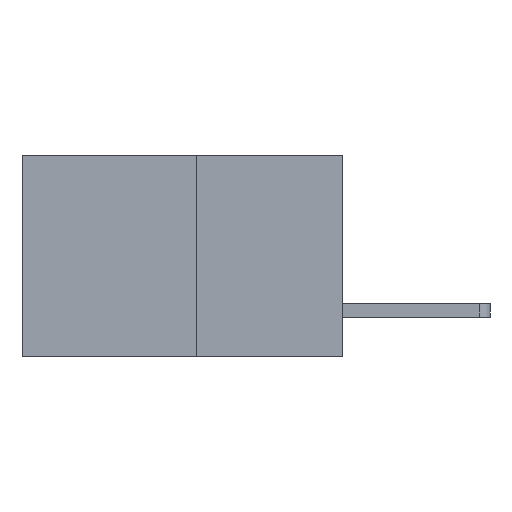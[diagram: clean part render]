
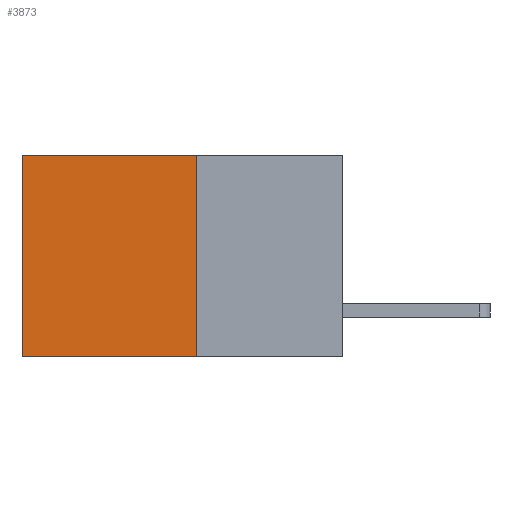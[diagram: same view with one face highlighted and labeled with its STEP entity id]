
A CAD part, left-side view. The second image highlights one B-rep face of the part: STEP entity #3873.
In plain terms, the highlighted planar face has unit normal (-1, 0, 0).
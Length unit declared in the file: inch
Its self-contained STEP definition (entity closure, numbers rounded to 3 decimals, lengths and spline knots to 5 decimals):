
#268 = VERTEX_POINT ( 'NONE', #2553 ) ;
#429 = LINE ( 'NONE', #6060, #4109 ) ;
#767 = LINE ( 'NONE', #8134, #6339 ) ;
#948 = ORIENTED_EDGE ( 'NONE', *, *, #2649, .T. ) ;
#991 = VECTOR ( 'NONE', #4728, 39.37008 ) ;
#1065 = ORIENTED_EDGE ( 'NONE', *, *, #2760, .T. ) ;
#1213 = ORIENTED_EDGE ( 'NONE', *, *, #8194, .F. ) ;
#1446 = VERTEX_POINT ( 'NONE', #3208 ) ;
#1551 = LINE ( 'NONE', #8164, #8953 ) ;
#2466 = EDGE_CURVE ( 'NONE', #268, #2572, #1551, .T. ) ;
#2553 = CARTESIAN_POINT ( 'NONE',  ( 0.277, 0.27, 0. ) ) ;
#2572 = VERTEX_POINT ( 'NONE', #7183 ) ;
#2649 = EDGE_CURVE ( 'NONE', #268, #1446, #429, .T. ) ;
#2760 = EDGE_CURVE ( 'NONE', #1446, #2761, #6790, .T. ) ;
#2761 = VERTEX_POINT ( 'NONE', #4672 ) ;
#3208 = CARTESIAN_POINT ( 'NONE',  ( 0.277, 0.59, 0. ) ) ;
#3741 = ORIENTED_EDGE ( 'NONE', *, *, #2466, .F. ) ;
#3873 = ADVANCED_FACE ( 'NONE', ( #4999 ), #4704, .F. ) ;
#3883 = DIRECTION ( 'NONE',  ( 0., 1., 0. ) ) ;
#4109 = VECTOR ( 'NONE', #6107, 39.37008 ) ;
#4413 = DIRECTION ( 'NONE',  ( 0., 0., -1. ) ) ;
#4636 = DIRECTION ( 'NONE',  ( 1., 0., 0. ) ) ;
#4670 = CARTESIAN_POINT ( 'NONE',  ( 0.277, 0.27, -0.37 ) ) ;
#4672 = CARTESIAN_POINT ( 'NONE',  ( 0.277, 0.59, -0.37 ) ) ;
#4682 = CARTESIAN_POINT ( 'NONE',  ( 0.277, 0.59, -0.37 ) ) ;
#4697 = AXIS2_PLACEMENT_3D ( 'NONE', #4670, #4636, #4413 ) ;
#4704 = PLANE ( 'NONE',  #4697 ) ;
#4728 = DIRECTION ( 'NONE',  ( 0., 0., -1. ) ) ;
#4845 = EDGE_LOOP ( 'NONE', ( #1065, #1213, #3741, #948 ) ) ;
#4999 = FACE_OUTER_BOUND ( 'NONE', #4845, .T. ) ;
#6060 = CARTESIAN_POINT ( 'NONE',  ( 0.277, 0.27, 0. ) ) ;
#6107 = DIRECTION ( 'NONE',  ( 0., 1., 0. ) ) ;
#6339 = VECTOR ( 'NONE', #3883, 39.37008 ) ;
#6790 = LINE ( 'NONE', #4682, #991 ) ;
#7183 = CARTESIAN_POINT ( 'NONE',  ( 0.277, 0.27, -0.37 ) ) ;
#7360 = DIRECTION ( 'NONE',  ( 0., 0., -1. ) ) ;
#8134 = CARTESIAN_POINT ( 'NONE',  ( 0.277, 0.27, -0.37 ) ) ;
#8164 = CARTESIAN_POINT ( 'NONE',  ( 0.277, 0.27, -0.37 ) ) ;
#8194 = EDGE_CURVE ( 'NONE', #2572, #2761, #767, .T. ) ;
#8953 = VECTOR ( 'NONE', #7360, 39.37008 ) ;
